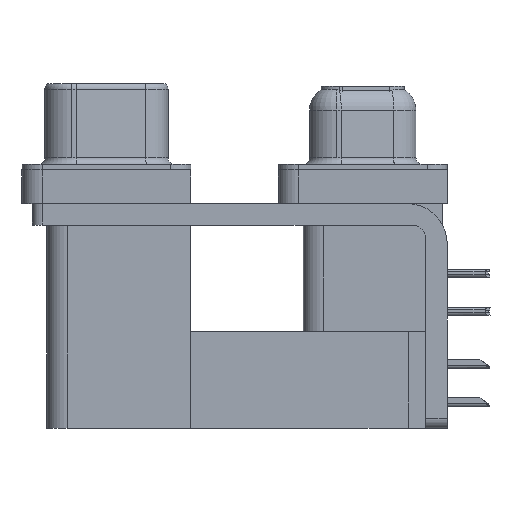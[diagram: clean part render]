
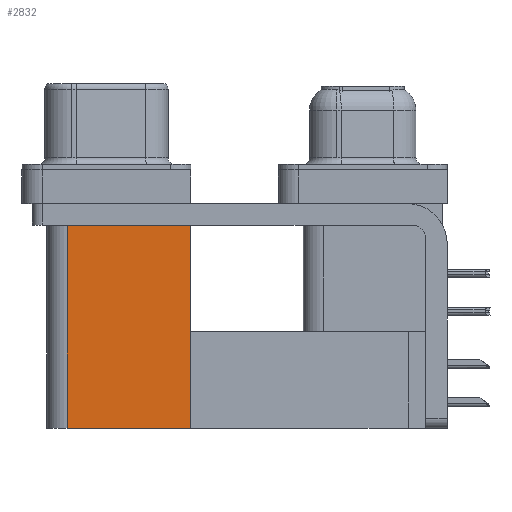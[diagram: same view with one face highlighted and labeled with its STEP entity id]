
A CAD part, left-side view. The second image highlights one B-rep face of the part: STEP entity #2832.
In plain terms, the highlighted planar face has unit normal (-1, 0, 0).
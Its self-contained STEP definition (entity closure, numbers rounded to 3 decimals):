
#1634 = DIRECTION ( 'NONE',  ( 0., 1., 0. ) ) ;
#2637 = ORIENTED_EDGE ( 'NONE', *, *, #4106, .F. ) ;
#2832 = ADVANCED_FACE ( 'NONE', ( #25503 ), #42651, .F. ) ;
#3543 = VERTEX_POINT ( 'NONE', #37668 ) ;
#4106 = EDGE_CURVE ( 'NONE', #33000, #31308, #4200, .T. ) ;
#4200 = LINE ( 'NONE', #31364, #39547 ) ;
#6778 = ORIENTED_EDGE ( 'NONE', *, *, #23203, .T. ) ;
#6847 = CARTESIAN_POINT ( 'NONE',  ( 3.765, 21.975, -19.2 ) ) ;
#7743 = ORIENTED_EDGE ( 'NONE', *, *, #33411, .F. ) ;
#11678 = CARTESIAN_POINT ( 'NONE',  ( 3.765, 12.775, -19.2 ) ) ;
#12020 = EDGE_CURVE ( 'NONE', #41597, #3543, #16205, .T. ) ;
#14350 = DIRECTION ( 'NONE',  ( 0., 1., 0. ) ) ;
#14418 = DIRECTION ( 'NONE',  ( 0., 0., 1. ) ) ;
#15976 = CARTESIAN_POINT ( 'NONE',  ( 3.765, 12.775, -19.2 ) ) ;
#16205 = LINE ( 'NONE', #15976, #37344 ) ;
#18990 = CARTESIAN_POINT ( 'NONE',  ( 3.765, 12.775, -2.5 ) ) ;
#19249 = CARTESIAN_POINT ( 'NONE',  ( 3.765, 12.775, -19.2 ) ) ;
#19756 = CARTESIAN_POINT ( 'NONE',  ( 3.765, 21.975, -2.5 ) ) ;
#20638 = ORIENTED_EDGE ( 'NONE', *, *, #12020, .T. ) ;
#22694 = DIRECTION ( 'NONE',  ( 0., 0., 1. ) ) ;
#23203 = EDGE_CURVE ( 'NONE', #3543, #31308, #35928, .T. ) ;
#25503 = FACE_OUTER_BOUND ( 'NONE', #31800, .T. ) ;
#27127 = CARTESIAN_POINT ( 'NONE',  ( 3.765, 12.775, -19.2 ) ) ;
#28347 = VECTOR ( 'NONE', #14350, 1000. ) ;
#31308 = VERTEX_POINT ( 'NONE', #19756 ) ;
#31364 = CARTESIAN_POINT ( 'NONE',  ( 3.765, 21.975, -19.2 ) ) ;
#31800 = EDGE_LOOP ( 'NONE', ( #6778, #2637, #7743, #20638 ) ) ;
#33000 = VERTEX_POINT ( 'NONE', #6847 ) ;
#33411 = EDGE_CURVE ( 'NONE', #41597, #33000, #41317, .T. ) ;
#34136 = AXIS2_PLACEMENT_3D ( 'NONE', #19249, #39304, #35737 ) ;
#35737 = DIRECTION ( 'NONE',  ( 0., 0., -1. ) ) ;
#35928 = LINE ( 'NONE', #18990, #42347 ) ;
#37344 = VECTOR ( 'NONE', #22694, 1000. ) ;
#37668 = CARTESIAN_POINT ( 'NONE',  ( 3.765, 12.775, -2.5 ) ) ;
#39304 = DIRECTION ( 'NONE',  ( 1., 0., 0. ) ) ;
#39547 = VECTOR ( 'NONE', #14418, 1000. ) ;
#41317 = LINE ( 'NONE', #11678, #28347 ) ;
#41597 = VERTEX_POINT ( 'NONE', #27127 ) ;
#42347 = VECTOR ( 'NONE', #1634, 1000. ) ;
#42651 = PLANE ( 'NONE',  #34136 ) ;
